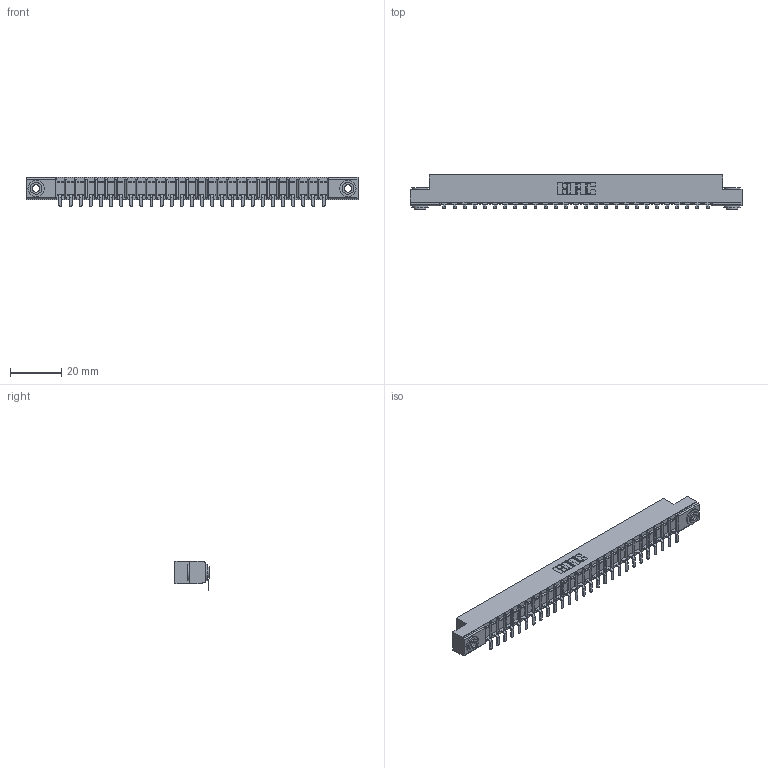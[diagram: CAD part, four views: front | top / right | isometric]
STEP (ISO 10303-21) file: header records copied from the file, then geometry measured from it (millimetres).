
FILE_DESCRIPTION (( 'STEP AP203' ), '1' );
FILE_NAME ('307-027-553-103.STEP', '2018-08-04T15:31:28', ( '' ), ( '' ), 'SwSTEP 2.0', 'SolidWorks 2016', '' );
FILE_SCHEMA (( 'CONFIG_CONTROL_DESIGN' ));
Length unit declared in the file: inch
Products named in the file (4): 307 Part_.156 Dia Mounting Holes; 307-290-002_553; 345-250-002_345-250-002-102; 307-027-553-103
Assembly tree (30 placements, depth 2):
  307-027-553-103
    307 Part_.156 Dia Mounting Holes
    307-290-002_553  x27
    345-250-002_345-250-002-102  x2
Bounding box: 130 x 13.36 x 11.51 mm (x, y, z)
Volume: 8585.9 mm3; surface area: 16146.5 mm2
Topology: 30 solids, 30 shells, 2304 faces, 7023 edges, 4602 vertices
Faces by surface type: plane 1363, cylinder 877, sphere 56, cone 8
Entity records: 26915 total; most frequent: CARTESIAN_POINT 4517, ORIENTED_EDGE 4498, DIRECTION 4411, EDGE_CURVE 2249, VECTOR 1707, LINE 1707, VERTEX_POINT 1458, AXIS2_PLACEMENT_3D 1352
